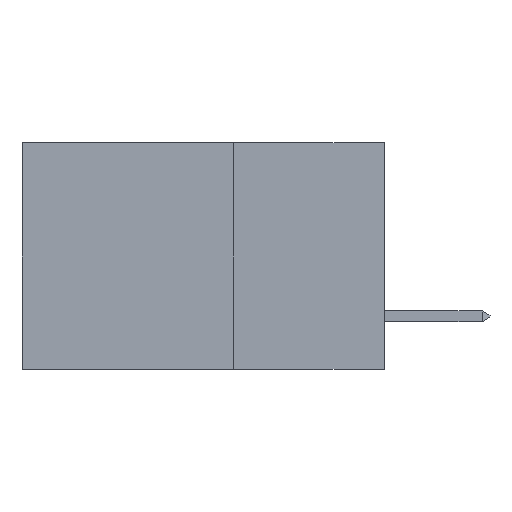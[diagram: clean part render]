
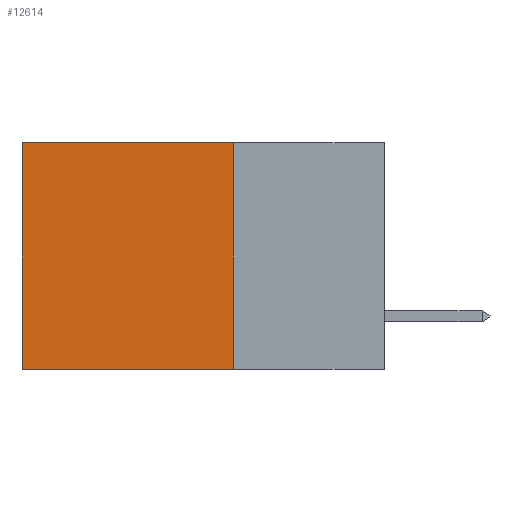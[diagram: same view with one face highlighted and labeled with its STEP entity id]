
A CAD part, left-side view. The second image highlights one B-rep face of the part: STEP entity #12614.
In plain terms, the highlighted planar face has unit normal (-1, 0, 0).
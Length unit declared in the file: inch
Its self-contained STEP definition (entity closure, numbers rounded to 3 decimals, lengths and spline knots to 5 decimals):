
#438 = ORIENTED_EDGE ( 'NONE', *, *, #3972, .T. ) ;
#450 = CARTESIAN_POINT ( 'NONE',  ( 0.2875, 0.6, 0. ) ) ;
#667 = EDGE_CURVE ( 'NONE', #5540, #10269, #885, .T. ) ;
#885 = LINE ( 'NONE', #10561, #9454 ) ;
#1226 = DIRECTION ( 'NONE',  ( 1., 0., 0. ) ) ;
#2219 = FACE_OUTER_BOUND ( 'NONE', #4891, .T. ) ;
#2937 = LINE ( 'NONE', #2998, #8486 ) ;
#2998 = CARTESIAN_POINT ( 'NONE',  ( 0.2875, 0.25, 0. ) ) ;
#3851 = VERTEX_POINT ( 'NONE', #6792 ) ;
#3972 = EDGE_CURVE ( 'NONE', #6830, #10269, #4643, .T. ) ;
#4083 = AXIS2_PLACEMENT_3D ( 'NONE', #7337, #1226, #7603 ) ;
#4138 = CARTESIAN_POINT ( 'NONE',  ( 0.2875, 0.6, -0.375 ) ) ;
#4206 = LINE ( 'NONE', #12402, #7395 ) ;
#4643 = LINE ( 'NONE', #7726, #12704 ) ;
#4891 = EDGE_LOOP ( 'NONE', ( #438, #11588, #12838, #12089 ) ) ;
#5441 = CARTESIAN_POINT ( 'NONE',  ( 0.2875, 0.25, -0.375 ) ) ;
#5540 = VERTEX_POINT ( 'NONE', #5441 ) ;
#6792 = CARTESIAN_POINT ( 'NONE',  ( 0.2875, 0.25, 0. ) ) ;
#6830 = VERTEX_POINT ( 'NONE', #450 ) ;
#7337 = CARTESIAN_POINT ( 'NONE',  ( 0.2875, 0.25, -0.375 ) ) ;
#7395 = VECTOR ( 'NONE', #13215, 39.37008 ) ;
#7603 = DIRECTION ( 'NONE',  ( 0., 0., -1. ) ) ;
#7726 = CARTESIAN_POINT ( 'NONE',  ( 0.2875, 0.6, -0.375 ) ) ;
#8486 = VECTOR ( 'NONE', #9196, 39.37008 ) ;
#9196 = DIRECTION ( 'NONE',  ( 0., 1., 0. ) ) ;
#9352 = DIRECTION ( 'NONE',  ( 0., 1., 0. ) ) ;
#9454 = VECTOR ( 'NONE', #9352, 39.37008 ) ;
#9639 = EDGE_CURVE ( 'NONE', #3851, #6830, #2937, .T. ) ;
#10217 = EDGE_CURVE ( 'NONE', #3851, #5540, #4206, .T. ) ;
#10269 = VERTEX_POINT ( 'NONE', #4138 ) ;
#10561 = CARTESIAN_POINT ( 'NONE',  ( 0.2875, 0.25, -0.375 ) ) ;
#10629 = PLANE ( 'NONE',  #4083 ) ;
#11588 = ORIENTED_EDGE ( 'NONE', *, *, #667, .F. ) ;
#11902 = DIRECTION ( 'NONE',  ( 0., 0., -1. ) ) ;
#12089 = ORIENTED_EDGE ( 'NONE', *, *, #9639, .T. ) ;
#12402 = CARTESIAN_POINT ( 'NONE',  ( 0.2875, 0.25, -0.375 ) ) ;
#12614 = ADVANCED_FACE ( 'NONE', ( #2219 ), #10629, .F. ) ;
#12704 = VECTOR ( 'NONE', #11902, 39.37008 ) ;
#12838 = ORIENTED_EDGE ( 'NONE', *, *, #10217, .F. ) ;
#13215 = DIRECTION ( 'NONE',  ( 0., 0., -1. ) ) ;
